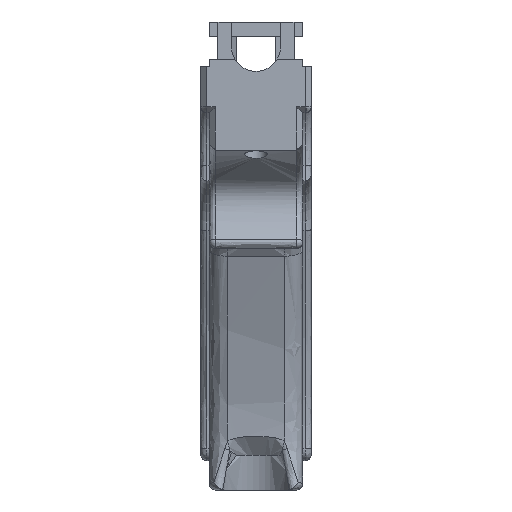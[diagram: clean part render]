
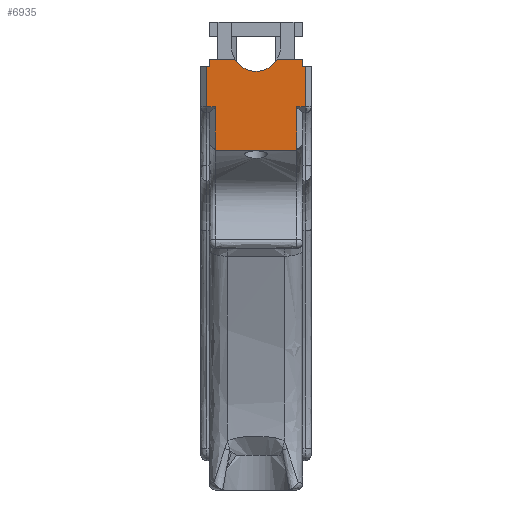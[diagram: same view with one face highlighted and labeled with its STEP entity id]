
A CAD part, front view. The second image highlights one B-rep face of the part: STEP entity #6935.
In plain terms, the highlighted planar face has unit normal (0, -1, 0).
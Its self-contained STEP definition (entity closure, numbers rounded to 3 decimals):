
#556=PLANE('',#7423);
#891=FACE_OUTER_BOUND('',#1284,.T.);
#1284=EDGE_LOOP('',(#6281,#6282,#6283,#6284,#6285,#6286,#6287,#6288,#6289,
#6290,#6291,#6292,#6293,#6294,#6295,#6296));
#1831=LINE('',#13939,#2473);
#1834=LINE('',#13945,#2476);
#1839=LINE('',#13957,#2481);
#1842=LINE('',#13962,#2484);
#1844=LINE('',#13966,#2486);
#1845=LINE('',#13968,#2487);
#1846=LINE('',#13971,#2488);
#1848=LINE('',#13975,#2490);
#1851=LINE('',#13980,#2493);
#1852=LINE('',#13982,#2494);
#1854=LINE('',#14007,#2496);
#1934=LINE('',#14583,#2576);
#1941=LINE('',#14597,#2583);
#1943=LINE('',#14601,#2585);
#1944=LINE('',#14602,#2586);
#2473=VECTOR('',#8665,10.);
#2476=VECTOR('',#8670,10.);
#2481=VECTOR('',#8681,10.);
#2484=VECTOR('',#8686,10.);
#2486=VECTOR('',#8690,10.);
#2487=VECTOR('',#8693,10.);
#2488=VECTOR('',#8696,10.);
#2490=VECTOR('',#8700,10.);
#2493=VECTOR('',#8705,10.);
#2494=VECTOR('',#8708,10.);
#2496=VECTOR('',#8714,10.);
#2576=VECTOR('',#8910,10.);
#2583=VECTOR('',#8921,10.);
#2585=VECTOR('',#8925,10.);
#2586=VECTOR('',#8926,10.);
#2758=CIRCLE('',#7352,4.2);
#3141=VERTEX_POINT('',#12261);
#3338=VERTEX_POINT('',#13936);
#3339=VERTEX_POINT('',#13938);
#3341=VERTEX_POINT('',#13944);
#3343=VERTEX_POINT('',#13950);
#3344=VERTEX_POINT('',#13952);
#3345=VERTEX_POINT('',#13956);
#3346=VERTEX_POINT('',#13960);
#3347=VERTEX_POINT('',#13964);
#3348=VERTEX_POINT('',#13970);
#3349=VERTEX_POINT('',#13974);
#3350=VERTEX_POINT('',#13978);
#3354=VERTEX_POINT('',#14006);
#3423=VERTEX_POINT('',#14582);
#3428=VERTEX_POINT('',#14595);
#3429=VERTEX_POINT('',#14600);
#4261=EDGE_CURVE('',#3339,#3338,#1831,.T.);
#4264=EDGE_CURVE('',#3339,#3341,#1834,.T.);
#4268=EDGE_CURVE('',#3344,#3343,#2758,.T.);
#4270=EDGE_CURVE('',#3344,#3345,#1839,.T.);
#4273=EDGE_CURVE('',#3345,#3346,#1842,.T.);
#4275=EDGE_CURVE('',#3347,#3346,#1844,.T.);
#4276=EDGE_CURVE('',#3347,#3141,#1845,.T.);
#4277=EDGE_CURVE('',#3141,#3348,#1846,.T.);
#4279=EDGE_CURVE('',#3348,#3349,#1848,.T.);
#4282=EDGE_CURVE('',#3349,#3350,#1851,.F.);
#4283=EDGE_CURVE('',#3338,#3350,#1852,.T.);
#4288=EDGE_CURVE('',#3341,#3354,#1854,.T.);
#4402=EDGE_CURVE('',#3423,#3343,#1934,.T.);
#4409=EDGE_CURVE('',#3428,#3423,#1941,.T.);
#4411=EDGE_CURVE('',#3428,#3429,#1943,.T.);
#4412=EDGE_CURVE('',#3354,#3429,#1944,.T.);
#6281=ORIENTED_EDGE('',*,*,#4283,.T.);
#6282=ORIENTED_EDGE('',*,*,#4282,.F.);
#6283=ORIENTED_EDGE('',*,*,#4279,.F.);
#6284=ORIENTED_EDGE('',*,*,#4277,.F.);
#6285=ORIENTED_EDGE('',*,*,#4276,.F.);
#6286=ORIENTED_EDGE('',*,*,#4275,.T.);
#6287=ORIENTED_EDGE('',*,*,#4273,.F.);
#6288=ORIENTED_EDGE('',*,*,#4270,.F.);
#6289=ORIENTED_EDGE('',*,*,#4268,.T.);
#6290=ORIENTED_EDGE('',*,*,#4402,.F.);
#6291=ORIENTED_EDGE('',*,*,#4409,.F.);
#6292=ORIENTED_EDGE('',*,*,#4411,.T.);
#6293=ORIENTED_EDGE('',*,*,#4412,.F.);
#6294=ORIENTED_EDGE('',*,*,#4288,.F.);
#6295=ORIENTED_EDGE('',*,*,#4264,.F.);
#6296=ORIENTED_EDGE('',*,*,#4261,.T.);
#6935=ADVANCED_FACE('',(#891),#556,.T.);
#7352=AXIS2_PLACEMENT_3D('',#13953,#8676,#8677);
#7423=AXIS2_PLACEMENT_3D('',#14599,#8923,#8924);
#8665=DIRECTION('',(0.707,0.,-0.707));
#8670=DIRECTION('',(0.,0.,1.));
#8676=DIRECTION('center_axis',(0.,1.,0.));
#8677=DIRECTION('ref_axis',(1.,0.,0.));
#8681=DIRECTION('',(1.,0.,0.));
#8686=DIRECTION('',(0.,0.,-1.));
#8690=DIRECTION('',(-1.,0.,0.));
#8693=DIRECTION('',(0.,0.,-1.));
#8696=DIRECTION('',(-1.,0.,0.));
#8700=DIRECTION('',(0.,0.,-1.));
#8705=DIRECTION('',(0.707,0.,0.707));
#8708=DIRECTION('',(1.,0.,0.));
#8714=DIRECTION('',(-1.,0.,0.));
#8910=DIRECTION('',(1.,0.,0.));
#8921=DIRECTION('',(0.,0.,1.));
#8923=DIRECTION('center_axis',(0.,-1.,0.));
#8924=DIRECTION('ref_axis',(0.,0.,-1.));
#8925=DIRECTION('',(-1.,0.,0.));
#8926=DIRECTION('',(0.,0.,1.));
#12261=CARTESIAN_POINT('',(16.4,-118.,-4.6));
#13936=CARTESIAN_POINT('',(1.057,-118.,-12.057));
#13938=CARTESIAN_POINT('',(1.,-118.,-12.));
#13939=CARTESIAN_POINT('',(-3.375,-118.,-7.625));
#13944=CARTESIAN_POINT('',(1.,-118.,-4.6));
#13945=CARTESIAN_POINT('',(1.,-118.,-7.95));
#13950=CARTESIAN_POINT('',(4.356,-118.,3.5));
#13952=CARTESIAN_POINT('',(11.544,-118.,3.5));
#13953=CARTESIAN_POINT('Origin',(7.95,-118.,5.673));
#13956=CARTESIAN_POINT('',(15.9,-118.,3.5));
#13957=CARTESIAN_POINT('',(0.,-118.,3.5));
#13960=CARTESIAN_POINT('',(15.9,-118.,2.25));
#13962=CARTESIAN_POINT('',(15.9,-118.,5.1));
#13964=CARTESIAN_POINT('',(16.4,-118.,2.25));
#13966=CARTESIAN_POINT('',(17.4,-118.,2.25));
#13968=CARTESIAN_POINT('',(16.4,-118.,0.413));
#13970=CARTESIAN_POINT('',(14.9,-118.,-4.6));
#13971=CARTESIAN_POINT('',(0.725,-118.,-4.6));
#13974=CARTESIAN_POINT('',(14.9,-118.,-12.));
#13975=CARTESIAN_POINT('',(14.9,-118.,5.1));
#13978=CARTESIAN_POINT('',(14.843,-118.,-12.057));
#13980=CARTESIAN_POINT('',(15.3,-118.,-11.6));
#13982=CARTESIAN_POINT('',(3.974,-118.,-12.057));
#14006=CARTESIAN_POINT('',(-0.5,-118.,-4.6));
#14007=CARTESIAN_POINT('',(0.725,-118.,-4.6));
#14582=CARTESIAN_POINT('',(0.,-118.,3.5));
#14583=CARTESIAN_POINT('',(0.,-118.,3.5));
#14595=CARTESIAN_POINT('',(0.,-118.,2.25));
#14597=CARTESIAN_POINT('',(0.,-118.,-7.95));
#14599=CARTESIAN_POINT('Origin',(0.,-118.,3.5));
#14600=CARTESIAN_POINT('',(-0.5,-118.,2.25));
#14601=CARTESIAN_POINT('',(-1.5,-118.,2.25));
#14602=CARTESIAN_POINT('',(-0.5,-118.,0.413));
